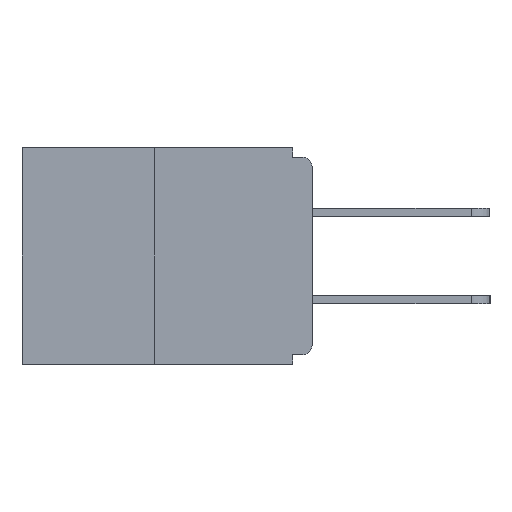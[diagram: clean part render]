
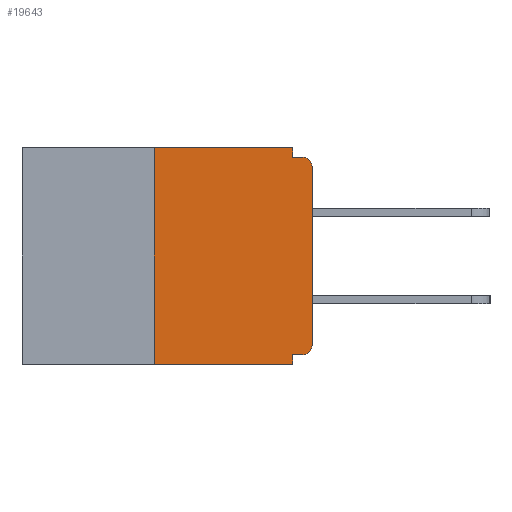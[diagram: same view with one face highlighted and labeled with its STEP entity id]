
A CAD part, left-side view. The second image highlights one B-rep face of the part: STEP entity #19643.
In plain terms, the highlighted planar face has unit normal (-1, 0, 0).
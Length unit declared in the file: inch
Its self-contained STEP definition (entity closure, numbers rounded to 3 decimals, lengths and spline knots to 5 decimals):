
#494 = DIRECTION ( 'NONE',  ( 1., 0., 0. ) ) ;
#1042 = DIRECTION ( 'NONE',  ( 0., -1., 0. ) ) ;
#1080 = CARTESIAN_POINT ( 'NONE',  ( 0., 0.031, -0.343 ) ) ;
#1391 = VECTOR ( 'NONE', #20172, 39.37008 ) ;
#1473 = CARTESIAN_POINT ( 'NONE',  ( 0., 0.031, 0. ) ) ;
#1708 = CARTESIAN_POINT ( 'NONE',  ( 0., 0.015, -0.313 ) ) ;
#1940 = EDGE_CURVE ( 'NONE', #21787, #10039, #6937, .T. ) ;
#2067 = ORIENTED_EDGE ( 'NONE', *, *, #11917, .F. ) ;
#2642 = DIRECTION ( 'NONE',  ( 0., -1., 0. ) ) ;
#2928 = CARTESIAN_POINT ( 'NONE',  ( 0., 0.031, -0.328 ) ) ;
#2941 = EDGE_CURVE ( 'NONE', #10161, #10039, #16654, .T. ) ;
#3526 = VERTEX_POINT ( 'NONE', #1473 ) ;
#3536 = EDGE_CURVE ( 'NONE', #12860, #11111, #5219, .T. ) ;
#3633 = CARTESIAN_POINT ( 'NONE',  ( 0., 0., -0.313 ) ) ;
#4098 = ORIENTED_EDGE ( 'NONE', *, *, #3536, .T. ) ;
#4099 = DIRECTION ( 'NONE',  ( 0., 0., -1. ) ) ;
#4402 = CARTESIAN_POINT ( 'NONE',  ( 0., 0., -0.328 ) ) ;
#4713 = CARTESIAN_POINT ( 'NONE',  ( 0., 0.015, -0.015 ) ) ;
#5219 = CIRCLE ( 'NONE', #5951, 0.015 ) ;
#5292 = LINE ( 'NONE', #19159, #21267 ) ;
#5843 = FACE_OUTER_BOUND ( 'NONE', #10428, .T. ) ;
#5951 = AXIS2_PLACEMENT_3D ( 'NONE', #1708, #16163, #22750 ) ;
#6385 = ORIENTED_EDGE ( 'NONE', *, *, #9725, .F. ) ;
#6425 = EDGE_CURVE ( 'NONE', #11111, #21787, #5292, .T. ) ;
#6686 = CARTESIAN_POINT ( 'NONE',  ( 0., 0.25, 0. ) ) ;
#6844 = CARTESIAN_POINT ( 'NONE',  ( 0., 0.46, -0.343 ) ) ;
#6875 = DIRECTION ( 'NONE',  ( 0., 0., -1. ) ) ;
#6937 = CIRCLE ( 'NONE', #9152, 0.015 ) ;
#8474 = LINE ( 'NONE', #6844, #20509 ) ;
#8496 = DIRECTION ( 'NONE',  ( -1., 0., 0. ) ) ;
#8523 = ORIENTED_EDGE ( 'NONE', *, *, #17005, .F. ) ;
#8632 = DIRECTION ( 'NONE',  ( 0., 0., 1. ) ) ;
#8986 = ORIENTED_EDGE ( 'NONE', *, *, #2941, .F. ) ;
#9005 = VECTOR ( 'NONE', #1042, 39.37008 ) ;
#9152 = AXIS2_PLACEMENT_3D ( 'NONE', #17156, #8496, #6875 ) ;
#9725 = EDGE_CURVE ( 'NONE', #12860, #19744, #20236, .T. ) ;
#9910 = LINE ( 'NONE', #15215, #14221 ) ;
#10039 = VERTEX_POINT ( 'NONE', #4713 ) ;
#10090 = EDGE_CURVE ( 'NONE', #3526, #10161, #9910, .T. ) ;
#10161 = VERTEX_POINT ( 'NONE', #15112 ) ;
#10366 = LINE ( 'NONE', #15558, #12507 ) ;
#10428 = EDGE_LOOP ( 'NONE', ( #2067, #21247, #13342, #8523, #6385, #4098, #20653, #18273, #8986, #18575 ) ) ;
#11111 = VERTEX_POINT ( 'NONE', #3633 ) ;
#11367 = CARTESIAN_POINT ( 'NONE',  ( 0., 0.25, -0.343 ) ) ;
#11440 = DIRECTION ( 'NONE',  ( 0., 1., 0. ) ) ;
#11917 = EDGE_CURVE ( 'NONE', #12030, #3526, #18378, .T. ) ;
#12030 = VERTEX_POINT ( 'NONE', #6686 ) ;
#12507 = VECTOR ( 'NONE', #15453, 39.37008 ) ;
#12860 = VERTEX_POINT ( 'NONE', #14470 ) ;
#12889 = PLANE ( 'NONE',  #15613 ) ;
#12947 = CARTESIAN_POINT ( 'NONE',  ( 0., 0., -0.03 ) ) ;
#13342 = ORIENTED_EDGE ( 'NONE', *, *, #22566, .T. ) ;
#13607 = DIRECTION ( 'NONE',  ( 0., 0., -1. ) ) ;
#14221 = VECTOR ( 'NONE', #13607, 39.37008 ) ;
#14470 = CARTESIAN_POINT ( 'NONE',  ( 0., 0.015, -0.328 ) ) ;
#14684 = VECTOR ( 'NONE', #2642, 39.37008 ) ;
#14897 = CARTESIAN_POINT ( 'NONE',  ( 0., 0.46, 0. ) ) ;
#14967 = LINE ( 'NONE', #1080, #1391 ) ;
#15112 = CARTESIAN_POINT ( 'NONE',  ( 0., 0.031, -0.015 ) ) ;
#15215 = CARTESIAN_POINT ( 'NONE',  ( 0., 0.031, 0. ) ) ;
#15453 = DIRECTION ( 'NONE',  ( 0., 0., 1. ) ) ;
#15558 = CARTESIAN_POINT ( 'NONE',  ( 0., 0.25, 0. ) ) ;
#15613 = AXIS2_PLACEMENT_3D ( 'NONE', #19934, #494, #4099 ) ;
#16163 = DIRECTION ( 'NONE',  ( -1., 0., 0. ) ) ;
#16181 = VERTEX_POINT ( 'NONE', #11367 ) ;
#16654 = LINE ( 'NONE', #16886, #9005 ) ;
#16753 = EDGE_CURVE ( 'NONE', #16181, #12030, #10366, .T. ) ;
#16886 = CARTESIAN_POINT ( 'NONE',  ( 0., 0., -0.015 ) ) ;
#17005 = EDGE_CURVE ( 'NONE', #19744, #19526, #14967, .T. ) ;
#17156 = CARTESIAN_POINT ( 'NONE',  ( 0., 0.015, -0.03 ) ) ;
#17476 = DIRECTION ( 'NONE',  ( 0., -1., 0. ) ) ;
#18273 = ORIENTED_EDGE ( 'NONE', *, *, #1940, .T. ) ;
#18378 = LINE ( 'NONE', #14897, #14684 ) ;
#18575 = ORIENTED_EDGE ( 'NONE', *, *, #10090, .F. ) ;
#19159 = CARTESIAN_POINT ( 'NONE',  ( 0., 0., 0. ) ) ;
#19498 = CARTESIAN_POINT ( 'NONE',  ( 0., 0.031, -0.343 ) ) ;
#19526 = VERTEX_POINT ( 'NONE', #19498 ) ;
#19643 = ADVANCED_FACE ( 'NONE', ( #5843 ), #12889, .F. ) ;
#19744 = VERTEX_POINT ( 'NONE', #2928 ) ;
#19934 = CARTESIAN_POINT ( 'NONE',  ( 0., 0.46, 0. ) ) ;
#20172 = DIRECTION ( 'NONE',  ( 0., 0., -1. ) ) ;
#20236 = LINE ( 'NONE', #4402, #21601 ) ;
#20509 = VECTOR ( 'NONE', #17476, 39.37008 ) ;
#20653 = ORIENTED_EDGE ( 'NONE', *, *, #6425, .T. ) ;
#21247 = ORIENTED_EDGE ( 'NONE', *, *, #16753, .F. ) ;
#21267 = VECTOR ( 'NONE', #8632, 39.37008 ) ;
#21601 = VECTOR ( 'NONE', #11440, 39.37008 ) ;
#21787 = VERTEX_POINT ( 'NONE', #12947 ) ;
#22566 = EDGE_CURVE ( 'NONE', #16181, #19526, #8474, .T. ) ;
#22750 = DIRECTION ( 'NONE',  ( 0., 0., -1. ) ) ;
